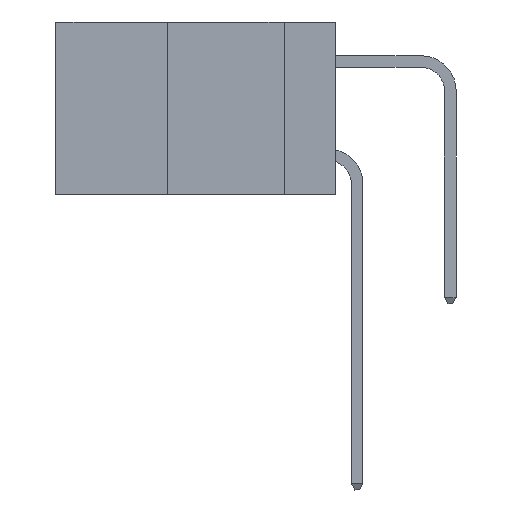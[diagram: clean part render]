
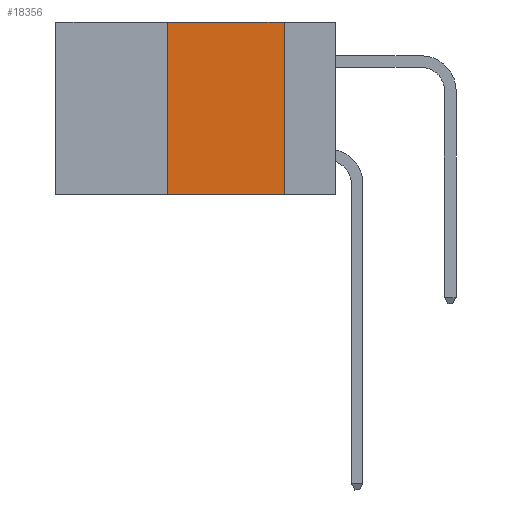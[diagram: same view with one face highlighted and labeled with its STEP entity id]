
A CAD part, left-side view. The second image highlights one B-rep face of the part: STEP entity #18356.
In plain terms, the highlighted planar face has unit normal (-1, 0, 0).
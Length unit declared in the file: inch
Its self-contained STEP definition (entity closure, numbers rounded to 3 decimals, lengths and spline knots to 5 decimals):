
#711 = VECTOR ( 'NONE', #2094, 39.37008 ) ;
#1071 = EDGE_CURVE ( 'NONE', #10724, #14380, #22267, .T. ) ;
#1254 = ORIENTED_EDGE ( 'NONE', *, *, #1071, .F. ) ;
#1511 = LINE ( 'NONE', #16059, #24652 ) ;
#2094 = DIRECTION ( 'NONE',  ( 0., -1., 0. ) ) ;
#3455 = LINE ( 'NONE', #23211, #711 ) ;
#4253 = ORIENTED_EDGE ( 'NONE', *, *, #20752, .F. ) ;
#4437 = DIRECTION ( 'NONE',  ( 0., 0., -1. ) ) ;
#5443 = ORIENTED_EDGE ( 'NONE', *, *, #7670, .F. ) ;
#5857 = EDGE_CURVE ( 'NONE', #10724, #9745, #3455, .T. ) ;
#7670 = EDGE_CURVE ( 'NONE', #14380, #16244, #1511, .T. ) ;
#9379 = FACE_OUTER_BOUND ( 'NONE', #24554, .T. ) ;
#9745 = VERTEX_POINT ( 'NONE', #11412 ) ;
#10724 = VERTEX_POINT ( 'NONE', #16650 ) ;
#10901 = DIRECTION ( 'NONE',  ( 1., 0., 0. ) ) ;
#11412 = CARTESIAN_POINT ( 'NONE',  ( 0., 0.11, -0.37 ) ) ;
#12913 = ORIENTED_EDGE ( 'NONE', *, *, #5857, .T. ) ;
#12943 = PLANE ( 'NONE',  #22654 ) ;
#13979 = DIRECTION ( 'NONE',  ( 0., -1., 0. ) ) ;
#14380 = VERTEX_POINT ( 'NONE', #20788 ) ;
#14653 = LINE ( 'NONE', #18184, #17622 ) ;
#15485 = CARTESIAN_POINT ( 'NONE',  ( 0., 0.36, 0. ) ) ;
#16059 = CARTESIAN_POINT ( 'NONE',  ( 0., 0.6, 0. ) ) ;
#16244 = VERTEX_POINT ( 'NONE', #21730 ) ;
#16650 = CARTESIAN_POINT ( 'NONE',  ( 0., 0.36, -0.37 ) ) ;
#17622 = VECTOR ( 'NONE', #4437, 39.37008 ) ;
#18184 = CARTESIAN_POINT ( 'NONE',  ( 0., 0.11, 0. ) ) ;
#18356 = ADVANCED_FACE ( 'NONE', ( #9379 ), #12943, .F. ) ;
#18980 = DIRECTION ( 'NONE',  ( 0., 0., 1. ) ) ;
#20379 = CARTESIAN_POINT ( 'NONE',  ( 0., 0.6, 0. ) ) ;
#20542 = DIRECTION ( 'NONE',  ( 0., 0., -1. ) ) ;
#20752 = EDGE_CURVE ( 'NONE', #16244, #9745, #14653, .T. ) ;
#20788 = CARTESIAN_POINT ( 'NONE',  ( 0., 0.36, 0. ) ) ;
#21675 = VECTOR ( 'NONE', #18980, 39.37008 ) ;
#21730 = CARTESIAN_POINT ( 'NONE',  ( 0., 0.11, 0. ) ) ;
#22267 = LINE ( 'NONE', #15485, #21675 ) ;
#22654 = AXIS2_PLACEMENT_3D ( 'NONE', #20379, #10901, #20542 ) ;
#23211 = CARTESIAN_POINT ( 'NONE',  ( 0., 0.6, -0.37 ) ) ;
#24554 = EDGE_LOOP ( 'NONE', ( #4253, #5443, #1254, #12913 ) ) ;
#24652 = VECTOR ( 'NONE', #13979, 39.37008 ) ;
